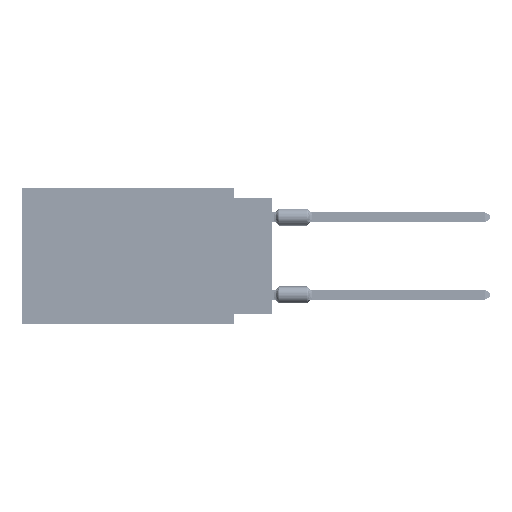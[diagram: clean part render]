
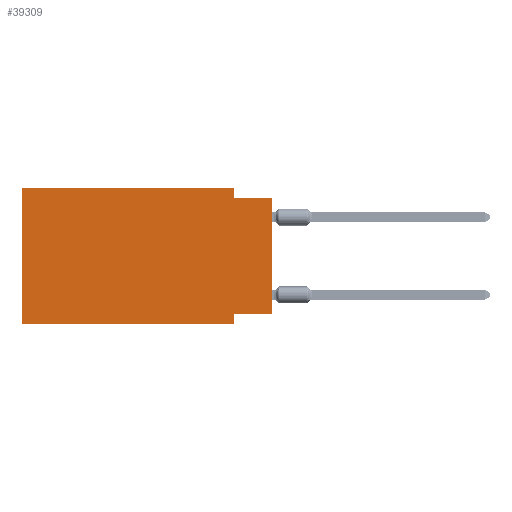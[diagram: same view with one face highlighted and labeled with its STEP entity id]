
A CAD part, left-side view. The second image highlights one B-rep face of the part: STEP entity #39309.
In plain terms, the highlighted planar face has unit normal (-1, 0, 0).
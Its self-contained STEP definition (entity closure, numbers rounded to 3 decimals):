
#167 = LINE ( 'NONE', #16220, #7433 ) ;
#2088 = CARTESIAN_POINT ( 'NONE',  ( 0., 2.54, 0. ) ) ;
#3004 = VERTEX_POINT ( 'NONE', #14492 ) ;
#6142 = EDGE_LOOP ( 'NONE', ( #69717, #58365, #56382, #7374, #46709, #53883, #18496, #69393 ) ) ;
#7374 = ORIENTED_EDGE ( 'NONE', *, *, #36326, .F. ) ;
#7433 = VECTOR ( 'NONE', #61408, 1000. ) ;
#8051 = VECTOR ( 'NONE', #40320, 1000. ) ;
#8083 = PLANE ( 'NONE',  #73209 ) ;
#13114 = DIRECTION ( 'NONE',  ( 0., -1., 0. ) ) ;
#13695 = CARTESIAN_POINT ( 'NONE',  ( 0., 16.383, 0. ) ) ;
#14421 = LINE ( 'NONE', #19668, #66209 ) ;
#14492 = CARTESIAN_POINT ( 'NONE',  ( 0., 2.54, -8.255 ) ) ;
#14586 = EDGE_CURVE ( 'NONE', #3004, #59072, #50687, .T. ) ;
#14719 = CARTESIAN_POINT ( 'NONE',  ( 0., 2.54, 0. ) ) ;
#15196 = VECTOR ( 'NONE', #13114, 1000. ) ;
#15981 = CARTESIAN_POINT ( 'NONE',  ( 0., 2.54, -8.89 ) ) ;
#16220 = CARTESIAN_POINT ( 'NONE',  ( 0., 16.383, 0. ) ) ;
#18496 = ORIENTED_EDGE ( 'NONE', *, *, #14586, .F. ) ;
#19305 = DIRECTION ( 'NONE',  ( 1., 0., 0. ) ) ;
#19668 = CARTESIAN_POINT ( 'NONE',  ( 0., 0., 0. ) ) ;
#20372 = EDGE_CURVE ( 'NONE', #37195, #57152, #65000, .T. ) ;
#20739 = EDGE_CURVE ( 'NONE', #32661, #37195, #53627, .T. ) ;
#21303 = CARTESIAN_POINT ( 'NONE',  ( 0., 16.383, 0. ) ) ;
#24408 = VECTOR ( 'NONE', #37361, 1000. ) ;
#26913 = LINE ( 'NONE', #21303, #24408 ) ;
#27199 = DIRECTION ( 'NONE',  ( 0., 1., 0. ) ) ;
#29796 = CARTESIAN_POINT ( 'NONE',  ( 0., 16.383, 0. ) ) ;
#30146 = FACE_OUTER_BOUND ( 'NONE', #6142, .T. ) ;
#30822 = CARTESIAN_POINT ( 'NONE',  ( 0., 2.54, -0.635 ) ) ;
#32661 = VERTEX_POINT ( 'NONE', #14719 ) ;
#32864 = LINE ( 'NONE', #50415, #45704 ) ;
#34034 = VERTEX_POINT ( 'NONE', #56210 ) ;
#34258 = VECTOR ( 'NONE', #27199, 1000. ) ;
#36326 = EDGE_CURVE ( 'NONE', #50315, #32661, #167, .T. ) ;
#37195 = VERTEX_POINT ( 'NONE', #30822 ) ;
#37361 = DIRECTION ( 'NONE',  ( 0., 0., 1. ) ) ;
#38019 = CARTESIAN_POINT ( 'NONE',  ( 0., 0., -8.255 ) ) ;
#39309 = ADVANCED_FACE ( 'NONE', ( #30146 ), #8083, .F. ) ;
#40320 = DIRECTION ( 'NONE',  ( 0., 0., -1. ) ) ;
#42447 = DIRECTION ( 'NONE',  ( 0., 0., 1. ) ) ;
#43643 = LINE ( 'NONE', #38019, #34258 ) ;
#45704 = VECTOR ( 'NONE', #67223, 1000. ) ;
#46289 = EDGE_CURVE ( 'NONE', #34034, #3004, #43643, .T. ) ;
#46709 = ORIENTED_EDGE ( 'NONE', *, *, #69946, .F. ) ;
#47318 = DIRECTION ( 'NONE',  ( 0., 0., -1. ) ) ;
#47768 = CARTESIAN_POINT ( 'NONE',  ( 0., 16.383, -8.89 ) ) ;
#50315 = VERTEX_POINT ( 'NONE', #13695 ) ;
#50415 = CARTESIAN_POINT ( 'NONE',  ( 0., 16.383, -8.89 ) ) ;
#50687 = LINE ( 'NONE', #73456, #56571 ) ;
#53627 = LINE ( 'NONE', #2088, #8051 ) ;
#53883 = ORIENTED_EDGE ( 'NONE', *, *, #66249, .T. ) ;
#55639 = EDGE_CURVE ( 'NONE', #34034, #57152, #14421, .T. ) ;
#56210 = CARTESIAN_POINT ( 'NONE',  ( 0., 0., -8.255 ) ) ;
#56382 = ORIENTED_EDGE ( 'NONE', *, *, #20739, .F. ) ;
#56571 = VECTOR ( 'NONE', #72333, 1000. ) ;
#57152 = VERTEX_POINT ( 'NONE', #58099 ) ;
#57838 = VERTEX_POINT ( 'NONE', #47768 ) ;
#58099 = CARTESIAN_POINT ( 'NONE',  ( 0., 0., -0.635 ) ) ;
#58365 = ORIENTED_EDGE ( 'NONE', *, *, #20372, .F. ) ;
#59072 = VERTEX_POINT ( 'NONE', #15981 ) ;
#61408 = DIRECTION ( 'NONE',  ( 0., -1., 0. ) ) ;
#64279 = CARTESIAN_POINT ( 'NONE',  ( 0., 0., -0.635 ) ) ;
#65000 = LINE ( 'NONE', #64279, #15196 ) ;
#66209 = VECTOR ( 'NONE', #42447, 1000. ) ;
#66249 = EDGE_CURVE ( 'NONE', #57838, #59072, #32864, .T. ) ;
#67223 = DIRECTION ( 'NONE',  ( 0., -1., 0. ) ) ;
#69393 = ORIENTED_EDGE ( 'NONE', *, *, #46289, .F. ) ;
#69717 = ORIENTED_EDGE ( 'NONE', *, *, #55639, .T. ) ;
#69946 = EDGE_CURVE ( 'NONE', #57838, #50315, #26913, .T. ) ;
#72333 = DIRECTION ( 'NONE',  ( 0., 0., -1. ) ) ;
#73209 = AXIS2_PLACEMENT_3D ( 'NONE', #29796, #19305, #47318 ) ;
#73456 = CARTESIAN_POINT ( 'NONE',  ( 0., 2.54, -8.89 ) ) ;
